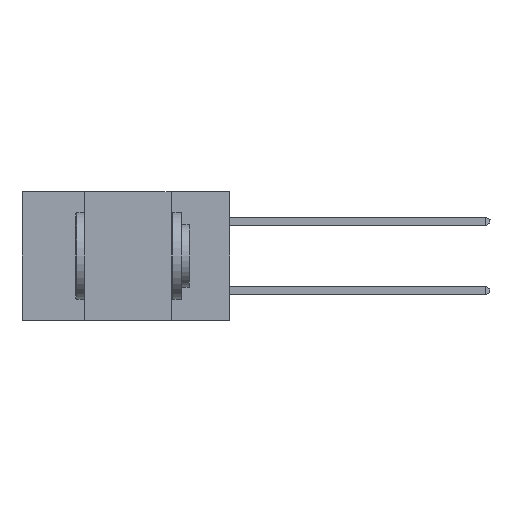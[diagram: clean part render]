
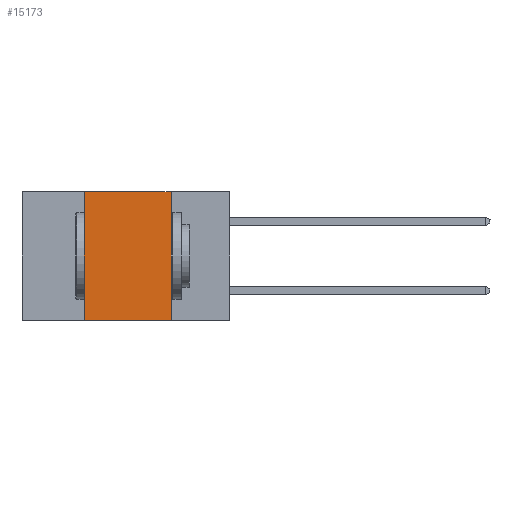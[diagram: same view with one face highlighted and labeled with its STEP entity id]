
A CAD part, left-side view. The second image highlights one B-rep face of the part: STEP entity #15173.
In plain terms, the highlighted planar face has unit normal (-1, 0, 0).
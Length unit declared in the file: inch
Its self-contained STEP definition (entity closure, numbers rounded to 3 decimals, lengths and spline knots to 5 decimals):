
#218 = DIRECTION ( 'NONE',  ( 0., 0., 1. ) ) ;
#996 = LINE ( 'NONE', #3928, #19158 ) ;
#1224 = LINE ( 'NONE', #1813, #14103 ) ;
#1813 = CARTESIAN_POINT ( 'NONE',  ( 0., 0.6, -0.37 ) ) ;
#2156 = CARTESIAN_POINT ( 'NONE',  ( 0., 0.42, -0.37 ) ) ;
#2359 = ORIENTED_EDGE ( 'NONE', *, *, #10398, .F. ) ;
#2392 = VERTEX_POINT ( 'NONE', #2156 ) ;
#3731 = CARTESIAN_POINT ( 'NONE',  ( 0., 0.42, 0. ) ) ;
#3888 = VECTOR ( 'NONE', #14979, 39.37008 ) ;
#3928 = CARTESIAN_POINT ( 'NONE',  ( 0., 0.6, 0. ) ) ;
#4960 = PLANE ( 'NONE',  #18159 ) ;
#5917 = EDGE_CURVE ( 'NONE', #19673, #17529, #20169, .T. ) ;
#6592 = CARTESIAN_POINT ( 'NONE',  ( 0., 0.17, 0. ) ) ;
#6794 = EDGE_CURVE ( 'NONE', #2392, #17529, #1224, .T. ) ;
#8078 = CARTESIAN_POINT ( 'NONE',  ( 0., 0.17, 0. ) ) ;
#8260 = DIRECTION ( 'NONE',  ( 0., -1., 0. ) ) ;
#8432 = DIRECTION ( 'NONE',  ( 0., 0., -1. ) ) ;
#9006 = VERTEX_POINT ( 'NONE', #15145 ) ;
#10398 = EDGE_CURVE ( 'NONE', #2392, #9006, #15047, .T. ) ;
#10563 = VECTOR ( 'NONE', #218, 39.37008 ) ;
#11736 = EDGE_LOOP ( 'NONE', ( #17068, #13250, #2359, #16830 ) ) ;
#12389 = EDGE_CURVE ( 'NONE', #9006, #19673, #996, .T. ) ;
#12436 = FACE_OUTER_BOUND ( 'NONE', #11736, .T. ) ;
#13250 = ORIENTED_EDGE ( 'NONE', *, *, #12389, .F. ) ;
#14103 = VECTOR ( 'NONE', #8260, 39.37008 ) ;
#14979 = DIRECTION ( 'NONE',  ( 0., 0., -1. ) ) ;
#15047 = LINE ( 'NONE', #3731, #10563 ) ;
#15145 = CARTESIAN_POINT ( 'NONE',  ( 0., 0.42, 0. ) ) ;
#15173 = ADVANCED_FACE ( 'NONE', ( #12436 ), #4960, .F. ) ;
#15483 = DIRECTION ( 'NONE',  ( 0., -1., 0. ) ) ;
#16676 = DIRECTION ( 'NONE',  ( 1., 0., 0. ) ) ;
#16830 = ORIENTED_EDGE ( 'NONE', *, *, #6794, .T. ) ;
#17068 = ORIENTED_EDGE ( 'NONE', *, *, #5917, .F. ) ;
#17529 = VERTEX_POINT ( 'NONE', #19930 ) ;
#18159 = AXIS2_PLACEMENT_3D ( 'NONE', #18457, #16676, #8432 ) ;
#18457 = CARTESIAN_POINT ( 'NONE',  ( 0., 0.6, 0. ) ) ;
#19158 = VECTOR ( 'NONE', #15483, 39.37008 ) ;
#19673 = VERTEX_POINT ( 'NONE', #6592 ) ;
#19930 = CARTESIAN_POINT ( 'NONE',  ( 0., 0.17, -0.37 ) ) ;
#20169 = LINE ( 'NONE', #8078, #3888 ) ;
